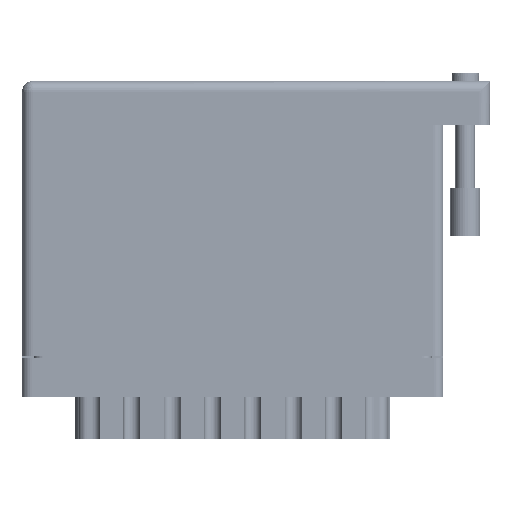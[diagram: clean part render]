
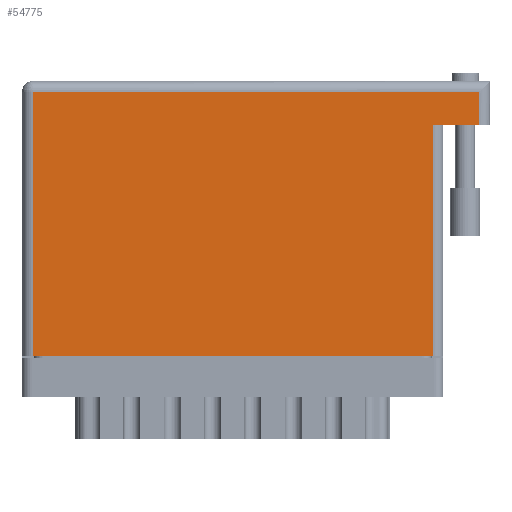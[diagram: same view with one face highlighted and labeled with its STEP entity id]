
A CAD part, front view. The second image highlights one B-rep face of the part: STEP entity #54775.
In plain terms, the highlighted face is planar.
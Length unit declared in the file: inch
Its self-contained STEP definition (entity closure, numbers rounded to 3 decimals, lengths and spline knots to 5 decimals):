
#33 = CARTESIAN_POINT ( 'NONE',  ( 0., 0., 0. ) ) ;
#2175 = ORIENTED_EDGE ( 'NONE', *, *, #16393, .F. ) ;
#6410 = VERTEX_POINT ( 'NONE', #33135 ) ;
#6872 = EDGE_CURVE ( 'NONE', #21010, #34339, #23406, .T. ) ;
#12361 = VECTOR ( 'NONE', #20448, 39.37008 ) ;
#12650 = DIRECTION ( 'NONE',  ( -1., 0., 0. ) ) ;
#13420 = AXIS2_PLACEMENT_3D ( 'NONE', #35292, #65429, #12650 ) ;
#13900 = LINE ( 'NONE', #15855, #55304 ) ;
#15323 = VECTOR ( 'NONE', #35550, 39.37008 ) ;
#15855 = CARTESIAN_POINT ( 'NONE',  ( 0.07, 0., 0. ) ) ;
#16393 = EDGE_CURVE ( 'NONE', #20012, #6410, #72203, .T. ) ;
#18839 = LINE ( 'NONE', #67254, #12361 ) ;
#20012 = VERTEX_POINT ( 'NONE', #64712 ) ;
#20448 = DIRECTION ( 'NONE',  ( 0., 1., 0. ) ) ;
#20890 = LINE ( 'NONE', #33, #15323 ) ;
#21010 = VERTEX_POINT ( 'NONE', #57689 ) ;
#21289 = DIRECTION ( 'NONE',  ( 0., -1., 0. ) ) ;
#22867 = ORIENTED_EDGE ( 'NONE', *, *, #27310, .T. ) ;
#23406 = LINE ( 'NONE', #46354, #69453 ) ;
#24935 = DIRECTION ( 'NONE',  ( -1., 0., 0. ) ) ;
#25666 = ORIENTED_EDGE ( 'NONE', *, *, #62325, .T. ) ;
#25694 = CARTESIAN_POINT ( 'NONE',  ( 3.018, 1.495, 0. ) ) ;
#27310 = EDGE_CURVE ( 'NONE', #34339, #31900, #13900, .T. ) ;
#28220 = ORIENTED_EDGE ( 'NONE', *, *, #37888, .T. ) ;
#30404 = FACE_OUTER_BOUND ( 'NONE', #32937, .T. ) ;
#30518 = ORIENTED_EDGE ( 'NONE', *, *, #6872, .T. ) ;
#30967 = DIRECTION ( 'NONE',  ( 0., 1., 0. ) ) ;
#31900 = VERTEX_POINT ( 'NONE', #73808 ) ;
#32937 = EDGE_LOOP ( 'NONE', ( #48316, #25666, #2175, #28220, #30518, #22867 ) ) ;
#33135 = CARTESIAN_POINT ( 'NONE',  ( 2.648, 1.495, 0. ) ) ;
#34339 = VERTEX_POINT ( 'NONE', #74545 ) ;
#35292 = CARTESIAN_POINT ( 'NONE',  ( 0., 1.775, 0. ) ) ;
#35550 = DIRECTION ( 'NONE',  ( 1., 0., 0. ) ) ;
#37888 = EDGE_CURVE ( 'NONE', #20012, #21010, #18839, .T. ) ;
#46354 = CARTESIAN_POINT ( 'NONE',  ( 0., 1.705, 0. ) ) ;
#46523 = EDGE_CURVE ( 'NONE', #31900, #63741, #20890, .T. ) ;
#46835 = PLANE ( 'NONE',  #13420 ) ;
#48316 = ORIENTED_EDGE ( 'NONE', *, *, #46523, .T. ) ;
#54649 = VECTOR ( 'NONE', #24935, 39.37008 ) ;
#54775 = ADVANCED_FACE ( 'NONE', ( #30404 ), #46835, .F. ) ;
#55304 = VECTOR ( 'NONE', #21289, 39.37008 ) ;
#57689 = CARTESIAN_POINT ( 'NONE',  ( 2.948, 1.705, 0. ) ) ;
#57826 = LINE ( 'NONE', #66720, #74386 ) ;
#62325 = EDGE_CURVE ( 'NONE', #63741, #6410, #57826, .T. ) ;
#63741 = VERTEX_POINT ( 'NONE', #70531 ) ;
#64712 = CARTESIAN_POINT ( 'NONE',  ( 2.948, 1.495, 0. ) ) ;
#65429 = DIRECTION ( 'NONE',  ( 0., 0., -1. ) ) ;
#66720 = CARTESIAN_POINT ( 'NONE',  ( 2.648, 1.495, 0. ) ) ;
#67254 = CARTESIAN_POINT ( 'NONE',  ( 2.948, 1.775, 0. ) ) ;
#69453 = VECTOR ( 'NONE', #70320, 39.37008 ) ;
#70320 = DIRECTION ( 'NONE',  ( -1., 0., 0. ) ) ;
#70531 = CARTESIAN_POINT ( 'NONE',  ( 2.648, 0., 0. ) ) ;
#72203 = LINE ( 'NONE', #25694, #54649 ) ;
#73808 = CARTESIAN_POINT ( 'NONE',  ( 0.07, 0., 0. ) ) ;
#74386 = VECTOR ( 'NONE', #30967, 39.37008 ) ;
#74545 = CARTESIAN_POINT ( 'NONE',  ( 0.07, 1.705, 0. ) ) ;
